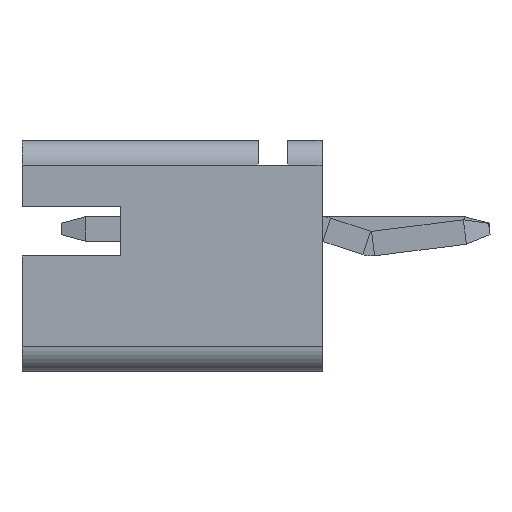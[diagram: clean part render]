
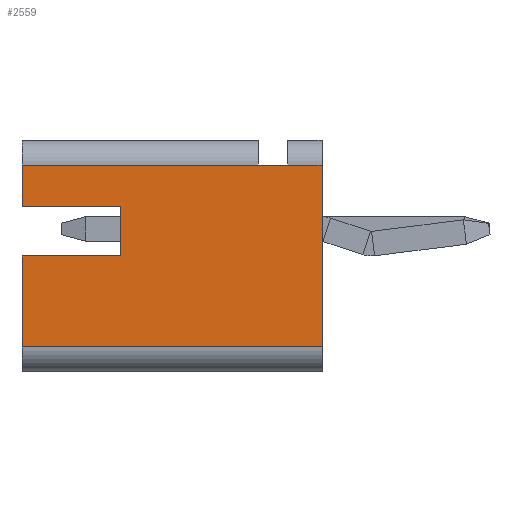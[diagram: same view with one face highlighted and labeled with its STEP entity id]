
A CAD part, left-side view. The second image highlights one B-rep face of the part: STEP entity #2559.
In plain terms, the highlighted planar face has unit normal (-1, 0, 0).
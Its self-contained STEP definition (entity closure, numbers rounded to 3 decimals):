
#12 = LINE ( 'NONE', #264, #780 ) ;
#185 = DIRECTION ( 'NONE',  ( 0., 0., 1. ) ) ;
#198 = VECTOR ( 'NONE', #2696, 1000. ) ;
#264 = CARTESIAN_POINT ( 'NONE',  ( -2., 6.1, 1.8 ) ) ;
#291 = LINE ( 'NONE', #2859, #1181 ) ;
#309 = DIRECTION ( 'NONE',  ( 0., 0., 1. ) ) ;
#314 = DIRECTION ( 'NONE',  ( 1., 0., 0. ) ) ;
#347 = DIRECTION ( 'NONE',  ( 0., -1., 0. ) ) ;
#480 = CARTESIAN_POINT ( 'NONE',  ( -2., 6.1, 0.45 ) ) ;
#615 = VERTEX_POINT ( 'NONE', #3468 ) ;
#702 = VERTEX_POINT ( 'NONE', #3858 ) ;
#714 = CARTESIAN_POINT ( 'NONE',  ( -2., 6.1, -2.4 ) ) ;
#765 = CARTESIAN_POINT ( 'NONE',  ( -2., 0., 1.3 ) ) ;
#780 = VECTOR ( 'NONE', #1321, 1000. ) ;
#808 = CARTESIAN_POINT ( 'NONE',  ( -2., 0., 1.8 ) ) ;
#904 = VERTEX_POINT ( 'NONE', #4513 ) ;
#967 = EDGE_CURVE ( 'NONE', #2616, #2320, #4401, .T. ) ;
#979 = EDGE_CURVE ( 'NONE', #3775, #615, #2665, .T. ) ;
#1020 = DIRECTION ( 'NONE',  ( 0., 1., 0. ) ) ;
#1154 = DIRECTION ( 'NONE',  ( 0., 0., -1. ) ) ;
#1168 = DIRECTION ( 'NONE',  ( 0., -1., 0. ) ) ;
#1181 = VECTOR ( 'NONE', #347, 1000. ) ;
#1321 = DIRECTION ( 'NONE',  ( 0., 0., 1. ) ) ;
#1346 = VECTOR ( 'NONE', #309, 1000. ) ;
#1399 = PLANE ( 'NONE',  #3950 ) ;
#1433 = EDGE_CURVE ( 'NONE', #2616, #615, #3485, .T. ) ;
#1477 = LINE ( 'NONE', #1668, #2240 ) ;
#1668 = CARTESIAN_POINT ( 'NONE',  ( -2., 4.1, 0.45 ) ) ;
#1902 = CARTESIAN_POINT ( 'NONE',  ( -2., 6.1, -0.55 ) ) ;
#1916 = CARTESIAN_POINT ( 'NONE',  ( -2., 1.3, 1.3 ) ) ;
#1940 = EDGE_CURVE ( 'NONE', #702, #3201, #4818, .T. ) ;
#2240 = VECTOR ( 'NONE', #185, 1000. ) ;
#2290 = EDGE_CURVE ( 'NONE', #3775, #904, #4274, .T. ) ;
#2320 = VERTEX_POINT ( 'NONE', #4749 ) ;
#2446 = ORIENTED_EDGE ( 'NONE', *, *, #979, .F. ) ;
#2450 = EDGE_CURVE ( 'NONE', #3201, #904, #12, .T. ) ;
#2481 = VERTEX_POINT ( 'NONE', #4059 ) ;
#2559 = ADVANCED_FACE ( 'NONE', ( #2652 ), #1399, .F. ) ;
#2616 = VERTEX_POINT ( 'NONE', #765 ) ;
#2619 = ORIENTED_EDGE ( 'NONE', *, *, #1433, .T. ) ;
#2652 = FACE_OUTER_BOUND ( 'NONE', #2714, .T. ) ;
#2665 = LINE ( 'NONE', #4085, #2786 ) ;
#2696 = DIRECTION ( 'NONE',  ( 0., 1., 0. ) ) ;
#2700 = LINE ( 'NONE', #4789, #1346 ) ;
#2714 = EDGE_LOOP ( 'NONE', ( #4826, #3506, #3949, #2619, #2446, #4051, #4170, #2746, #3973, #4297 ) ) ;
#2746 = ORIENTED_EDGE ( 'NONE', *, *, #1940, .F. ) ;
#2786 = VECTOR ( 'NONE', #1168, 1000. ) ;
#2859 = CARTESIAN_POINT ( 'NONE',  ( -2., 6.1, -0.55 ) ) ;
#2882 = EDGE_CURVE ( 'NONE', #4117, #2320, #3245, .T. ) ;
#2894 = EDGE_CURVE ( 'NONE', #2481, #702, #1477, .T. ) ;
#2931 = CARTESIAN_POINT ( 'NONE',  ( -2., 0., 0. ) ) ;
#3019 = VECTOR ( 'NONE', #1020, 1000. ) ;
#3119 = EDGE_CURVE ( 'NONE', #4594, #2481, #291, .T. ) ;
#3137 = EDGE_CURVE ( 'NONE', #4117, #4594, #2700, .T. ) ;
#3201 = VERTEX_POINT ( 'NONE', #3314 ) ;
#3245 = LINE ( 'NONE', #4328, #3470 ) ;
#3259 = VECTOR ( 'NONE', #1154, 1000. ) ;
#3264 = DIRECTION ( 'NONE',  ( 0., 1., 0. ) ) ;
#3271 = CARTESIAN_POINT ( 'NONE',  ( -2., 0., 1.3 ) ) ;
#3281 = CARTESIAN_POINT ( 'NONE',  ( -2., 0., 1.3 ) ) ;
#3314 = CARTESIAN_POINT ( 'NONE',  ( -2., 6.1, 0.45 ) ) ;
#3468 = CARTESIAN_POINT ( 'NONE',  ( -2., 0.7, 1.3 ) ) ;
#3470 = VECTOR ( 'NONE', #4689, 1000. ) ;
#3485 = LINE ( 'NONE', #3281, #4217 ) ;
#3506 = ORIENTED_EDGE ( 'NONE', *, *, #2882, .T. ) ;
#3775 = VERTEX_POINT ( 'NONE', #1916 ) ;
#3858 = CARTESIAN_POINT ( 'NONE',  ( -2., 4.1, 0.45 ) ) ;
#3949 = ORIENTED_EDGE ( 'NONE', *, *, #967, .F. ) ;
#3950 = AXIS2_PLACEMENT_3D ( 'NONE', #2931, #314, #4093 ) ;
#3973 = ORIENTED_EDGE ( 'NONE', *, *, #2894, .F. ) ;
#4051 = ORIENTED_EDGE ( 'NONE', *, *, #2290, .T. ) ;
#4059 = CARTESIAN_POINT ( 'NONE',  ( -2., 4.1, -0.55 ) ) ;
#4085 = CARTESIAN_POINT ( 'NONE',  ( -2., 1.3, 1.3 ) ) ;
#4093 = DIRECTION ( 'NONE',  ( 0., 0., -1. ) ) ;
#4117 = VERTEX_POINT ( 'NONE', #714 ) ;
#4170 = ORIENTED_EDGE ( 'NONE', *, *, #2450, .F. ) ;
#4217 = VECTOR ( 'NONE', #3264, 1000. ) ;
#4274 = LINE ( 'NONE', #3271, #3019 ) ;
#4297 = ORIENTED_EDGE ( 'NONE', *, *, #3119, .F. ) ;
#4328 = CARTESIAN_POINT ( 'NONE',  ( -2., 0., -2.4 ) ) ;
#4401 = LINE ( 'NONE', #808, #3259 ) ;
#4513 = CARTESIAN_POINT ( 'NONE',  ( -2., 6.1, 1.3 ) ) ;
#4594 = VERTEX_POINT ( 'NONE', #1902 ) ;
#4689 = DIRECTION ( 'NONE',  ( 0., -1., 0. ) ) ;
#4749 = CARTESIAN_POINT ( 'NONE',  ( -2., 0., -2.4 ) ) ;
#4789 = CARTESIAN_POINT ( 'NONE',  ( -2., 6.1, -0.55 ) ) ;
#4818 = LINE ( 'NONE', #480, #198 ) ;
#4826 = ORIENTED_EDGE ( 'NONE', *, *, #3137, .F. ) ;
